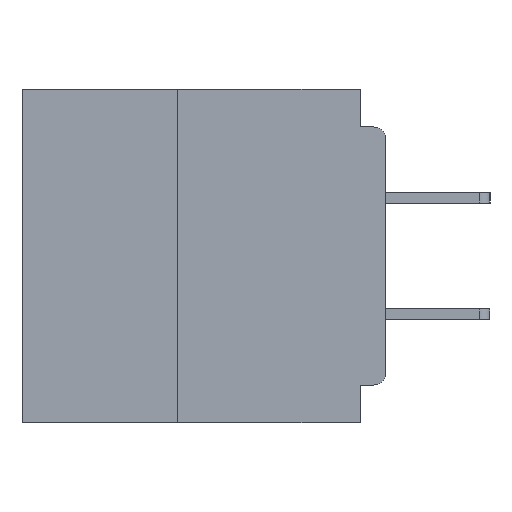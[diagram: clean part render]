
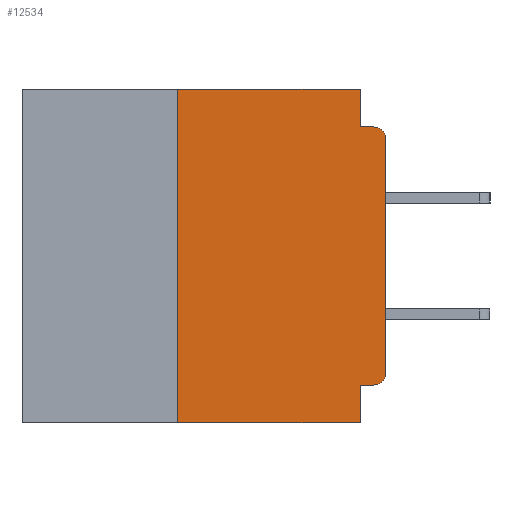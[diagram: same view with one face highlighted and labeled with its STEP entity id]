
A CAD part, left-side view. The second image highlights one B-rep face of the part: STEP entity #12534.
In plain terms, the highlighted planar face has unit normal (-1, 0, 0).
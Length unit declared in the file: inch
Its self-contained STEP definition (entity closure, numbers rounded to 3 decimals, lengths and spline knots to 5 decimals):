
#155 = VERTEX_POINT ( 'NONE', #57775 ) ;
#2172 = DIRECTION ( 'NONE',  ( 0., 0., 1. ) ) ;
#2711 = ORIENTED_EDGE ( 'NONE', *, *, #23852, .T. ) ;
#3161 = CIRCLE ( 'NONE', #24473, 0.015 ) ;
#3283 = VERTEX_POINT ( 'NONE', #51980 ) ;
#3458 = VECTOR ( 'NONE', #17367, 39.37008 ) ;
#3471 = ORIENTED_EDGE ( 'NONE', *, *, #20454, .F. ) ;
#3641 = EDGE_LOOP ( 'NONE', ( #7007, #2711, #9919, #3471, #4940, #52504, #47596, #7865, #43417, #52805 ) ) ;
#4846 = EDGE_CURVE ( 'NONE', #3283, #30456, #3161, .T. ) ;
#4940 = ORIENTED_EDGE ( 'NONE', *, *, #21583, .F. ) ;
#6386 = CARTESIAN_POINT ( 'NONE',  ( 0., 0.031, -0.4 ) ) ;
#7007 = ORIENTED_EDGE ( 'NONE', *, *, #10705, .T. ) ;
#7156 = LINE ( 'NONE', #15443, #53960 ) ;
#7408 = VERTEX_POINT ( 'NONE', #55222 ) ;
#7865 = ORIENTED_EDGE ( 'NONE', *, *, #50070, .F. ) ;
#9534 = CARTESIAN_POINT ( 'NONE',  ( 0., 0.015, -0.34 ) ) ;
#9787 = CARTESIAN_POINT ( 'NONE',  ( 0., 0.031, -0.355 ) ) ;
#9919 = ORIENTED_EDGE ( 'NONE', *, *, #55016, .F. ) ;
#10705 = EDGE_CURVE ( 'NONE', #30456, #7408, #17195, .T. ) ;
#10753 = DIRECTION ( 'NONE',  ( 0., -1., 0. ) ) ;
#10996 = DIRECTION ( 'NONE',  ( 0., 0., -1. ) ) ;
#11670 = EDGE_CURVE ( 'NONE', #3283, #25323, #36925, .T. ) ;
#12534 = ADVANCED_FACE ( 'NONE', ( #14924 ), #19263, .F. ) ;
#12543 = AXIS2_PLACEMENT_3D ( 'NONE', #42557, #15405, #47118 ) ;
#14121 = DIRECTION ( 'NONE',  ( 0., 0., -1. ) ) ;
#14924 = FACE_OUTER_BOUND ( 'NONE', #3641, .T. ) ;
#15405 = DIRECTION ( 'NONE',  ( -1., 0., 0. ) ) ;
#15443 = CARTESIAN_POINT ( 'NONE',  ( 0., 0.031, 0. ) ) ;
#17195 = LINE ( 'NONE', #46008, #27906 ) ;
#17367 = DIRECTION ( 'NONE',  ( 0., 1., 0. ) ) ;
#18578 = VERTEX_POINT ( 'NONE', #37363 ) ;
#19263 = PLANE ( 'NONE',  #31549 ) ;
#20454 = EDGE_CURVE ( 'NONE', #29120, #23774, #7156, .T. ) ;
#21583 = EDGE_CURVE ( 'NONE', #18578, #29120, #57909, .T. ) ;
#22909 = CARTESIAN_POINT ( 'NONE',  ( 0., 0.25, -0.4 ) ) ;
#23774 = VERTEX_POINT ( 'NONE', #32911 ) ;
#23852 = EDGE_CURVE ( 'NONE', #7408, #40924, #37872, .T. ) ;
#24473 = AXIS2_PLACEMENT_3D ( 'NONE', #9534, #41267, #14121 ) ;
#24897 = VERTEX_POINT ( 'NONE', #22909 ) ;
#25323 = VERTEX_POINT ( 'NONE', #9787 ) ;
#27596 = DIRECTION ( 'NONE',  ( 0., -1., 0. ) ) ;
#27906 = VECTOR ( 'NONE', #45817, 39.37008 ) ;
#28447 = DIRECTION ( 'NONE',  ( 0., 0., -1. ) ) ;
#29120 = VERTEX_POINT ( 'NONE', #46842 ) ;
#29273 = VECTOR ( 'NONE', #10996, 39.37008 ) ;
#30456 = VERTEX_POINT ( 'NONE', #56336 ) ;
#30743 = VECTOR ( 'NONE', #52976, 39.37008 ) ;
#31549 = AXIS2_PLACEMENT_3D ( 'NONE', #50908, #55434, #28447 ) ;
#32911 = CARTESIAN_POINT ( 'NONE',  ( 0., 0.031, -0.045 ) ) ;
#33423 = CARTESIAN_POINT ( 'NONE',  ( 0., 0.437, 0. ) ) ;
#36641 = CARTESIAN_POINT ( 'NONE',  ( 0., 0., -0.045 ) ) ;
#36925 = LINE ( 'NONE', #44536, #3458 ) ;
#37363 = CARTESIAN_POINT ( 'NONE',  ( 0., 0.25, 0. ) ) ;
#37872 = CIRCLE ( 'NONE', #12543, 0.015 ) ;
#38011 = EDGE_CURVE ( 'NONE', #24897, #18578, #52515, .T. ) ;
#39620 = EDGE_CURVE ( 'NONE', #24897, #155, #54736, .T. ) ;
#40011 = CARTESIAN_POINT ( 'NONE',  ( 0., 0.015, -0.045 ) ) ;
#40499 = VECTOR ( 'NONE', #2172, 39.37008 ) ;
#40924 = VERTEX_POINT ( 'NONE', #40011 ) ;
#41267 = DIRECTION ( 'NONE',  ( -1., 0., 0. ) ) ;
#42557 = CARTESIAN_POINT ( 'NONE',  ( 0., 0.015, -0.06 ) ) ;
#42966 = CARTESIAN_POINT ( 'NONE',  ( 0., 0.25, -0.4 ) ) ;
#43417 = ORIENTED_EDGE ( 'NONE', *, *, #11670, .F. ) ;
#44536 = CARTESIAN_POINT ( 'NONE',  ( 0., 0., -0.355 ) ) ;
#45817 = DIRECTION ( 'NONE',  ( 0., 0., 1. ) ) ;
#45976 = VECTOR ( 'NONE', #10753, 39.37008 ) ;
#46008 = CARTESIAN_POINT ( 'NONE',  ( 0., 0., 0. ) ) ;
#46557 = VECTOR ( 'NONE', #27596, 39.37008 ) ;
#46842 = CARTESIAN_POINT ( 'NONE',  ( 0., 0.031, 0. ) ) ;
#47118 = DIRECTION ( 'NONE',  ( 0., 0., -1. ) ) ;
#47596 = ORIENTED_EDGE ( 'NONE', *, *, #39620, .T. ) ;
#48463 = CARTESIAN_POINT ( 'NONE',  ( 0., 0.437, -0.4 ) ) ;
#50070 = EDGE_CURVE ( 'NONE', #25323, #155, #53228, .T. ) ;
#50908 = CARTESIAN_POINT ( 'NONE',  ( 0., 0.437, 0. ) ) ;
#51980 = CARTESIAN_POINT ( 'NONE',  ( 0., 0.015, -0.355 ) ) ;
#52504 = ORIENTED_EDGE ( 'NONE', *, *, #38011, .F. ) ;
#52515 = LINE ( 'NONE', #42966, #40499 ) ;
#52805 = ORIENTED_EDGE ( 'NONE', *, *, #4846, .T. ) ;
#52976 = DIRECTION ( 'NONE',  ( 0., -1., 0. ) ) ;
#53228 = LINE ( 'NONE', #6386, #29273 ) ;
#53960 = VECTOR ( 'NONE', #56227, 39.37008 ) ;
#54736 = LINE ( 'NONE', #48463, #30743 ) ;
#55016 = EDGE_CURVE ( 'NONE', #23774, #40924, #58511, .T. ) ;
#55222 = CARTESIAN_POINT ( 'NONE',  ( 0., 0., -0.06 ) ) ;
#55434 = DIRECTION ( 'NONE',  ( 1., 0., 0. ) ) ;
#56227 = DIRECTION ( 'NONE',  ( 0., 0., -1. ) ) ;
#56336 = CARTESIAN_POINT ( 'NONE',  ( 0., 0., -0.34 ) ) ;
#57775 = CARTESIAN_POINT ( 'NONE',  ( 0., 0.031, -0.4 ) ) ;
#57909 = LINE ( 'NONE', #33423, #45976 ) ;
#58511 = LINE ( 'NONE', #36641, #46557 ) ;
